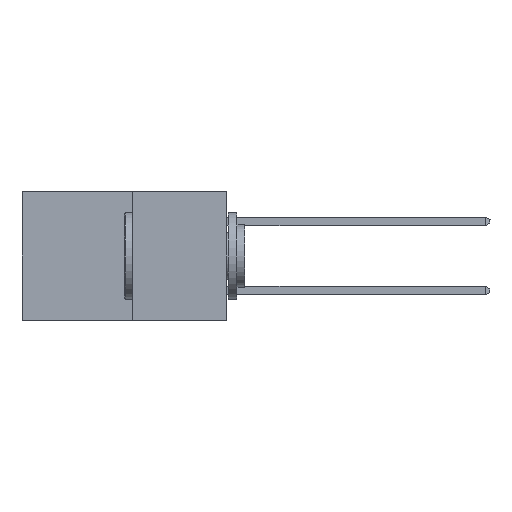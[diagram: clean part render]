
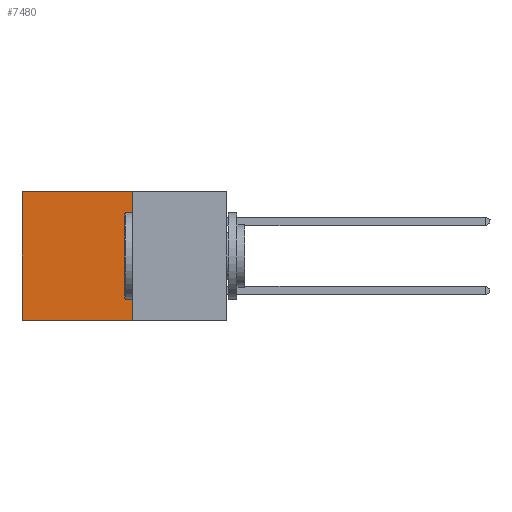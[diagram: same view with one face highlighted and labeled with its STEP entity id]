
A CAD part, left-side view. The second image highlights one B-rep face of the part: STEP entity #7480.
In plain terms, the highlighted planar face has unit normal (-1, 0, 0).
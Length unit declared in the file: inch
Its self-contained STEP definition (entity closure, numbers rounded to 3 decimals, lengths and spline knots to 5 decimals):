
#779 = CARTESIAN_POINT ( 'NONE',  ( 0.277, 0.27, -0.37 ) ) ;
#995 = EDGE_CURVE ( 'NONE', #2587, #8585, #9224, .T. ) ;
#1333 = EDGE_CURVE ( 'NONE', #10794, #8585, #4171, .T. ) ;
#1634 = VERTEX_POINT ( 'NONE', #6513 ) ;
#2587 = VERTEX_POINT ( 'NONE', #779 ) ;
#2893 = VECTOR ( 'NONE', #7685, 39.37008 ) ;
#3177 = EDGE_LOOP ( 'NONE', ( #7150, #13998, #3271, #8802 ) ) ;
#3271 = ORIENTED_EDGE ( 'NONE', *, *, #4521, .F. ) ;
#3294 = LINE ( 'NONE', #5399, #2893 ) ;
#4171 = LINE ( 'NONE', #14332, #12927 ) ;
#4521 = EDGE_CURVE ( 'NONE', #1634, #2587, #11489, .T. ) ;
#5110 = CARTESIAN_POINT ( 'NONE',  ( 0.277, 0.59, -0.37 ) ) ;
#5399 = CARTESIAN_POINT ( 'NONE',  ( 0.277, 0.27, 0. ) ) ;
#5417 = VECTOR ( 'NONE', #14322, 39.37008 ) ;
#6513 = CARTESIAN_POINT ( 'NONE',  ( 0.277, 0.27, 0. ) ) ;
#7150 = ORIENTED_EDGE ( 'NONE', *, *, #1333, .T. ) ;
#7480 = ADVANCED_FACE ( 'NONE', ( #12731 ), #14368, .F. ) ;
#7685 = DIRECTION ( 'NONE',  ( 0., 1., 0. ) ) ;
#8002 = CARTESIAN_POINT ( 'NONE',  ( 0.277, 0.59, 0. ) ) ;
#8585 = VERTEX_POINT ( 'NONE', #5110 ) ;
#8802 = ORIENTED_EDGE ( 'NONE', *, *, #9930, .T. ) ;
#9224 = LINE ( 'NONE', #13634, #9569 ) ;
#9569 = VECTOR ( 'NONE', #13716, 39.37008 ) ;
#9930 = EDGE_CURVE ( 'NONE', #1634, #10794, #3294, .T. ) ;
#10794 = VERTEX_POINT ( 'NONE', #8002 ) ;
#11192 = AXIS2_PLACEMENT_3D ( 'NONE', #14200, #14183, #14076 ) ;
#11489 = LINE ( 'NONE', #14344, #5417 ) ;
#12731 = FACE_OUTER_BOUND ( 'NONE', #3177, .T. ) ;
#12927 = VECTOR ( 'NONE', #14117, 39.37008 ) ;
#13634 = CARTESIAN_POINT ( 'NONE',  ( 0.277, 0.27, -0.37 ) ) ;
#13716 = DIRECTION ( 'NONE',  ( 0., 1., 0. ) ) ;
#13998 = ORIENTED_EDGE ( 'NONE', *, *, #995, .F. ) ;
#14076 = DIRECTION ( 'NONE',  ( 0., 0., -1. ) ) ;
#14117 = DIRECTION ( 'NONE',  ( 0., 0., -1. ) ) ;
#14183 = DIRECTION ( 'NONE',  ( 1., 0., 0. ) ) ;
#14200 = CARTESIAN_POINT ( 'NONE',  ( 0.277, 0.27, -0.37 ) ) ;
#14322 = DIRECTION ( 'NONE',  ( 0., 0., -1. ) ) ;
#14332 = CARTESIAN_POINT ( 'NONE',  ( 0.277, 0.59, -0.37 ) ) ;
#14344 = CARTESIAN_POINT ( 'NONE',  ( 0.277, 0.27, -0.37 ) ) ;
#14368 = PLANE ( 'NONE',  #11192 ) ;
